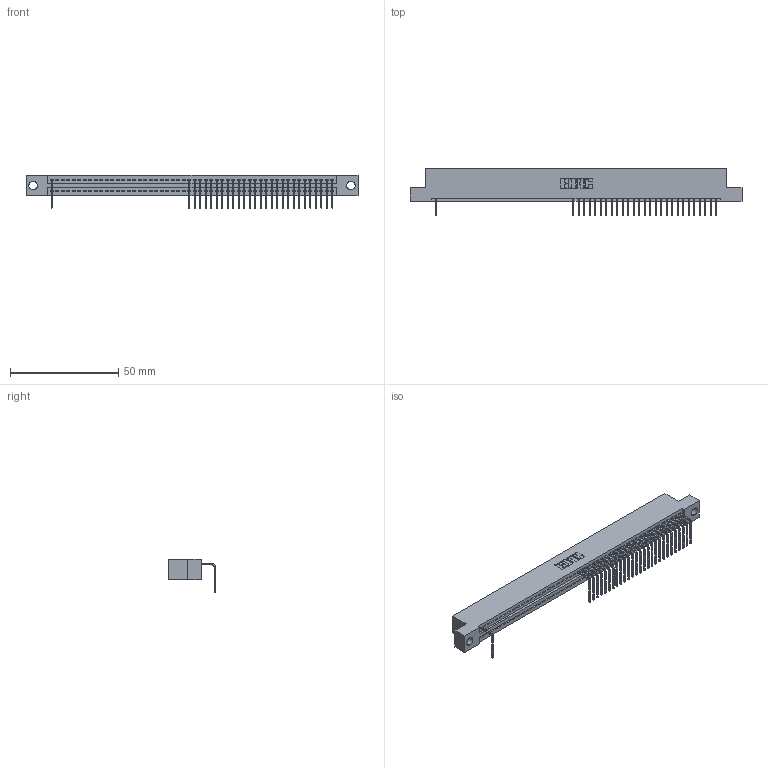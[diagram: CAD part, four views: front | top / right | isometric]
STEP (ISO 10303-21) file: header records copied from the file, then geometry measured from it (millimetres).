
FILE_DESCRIPTION (( 'STEP AP203' ), '1' );
FILE_NAME ('345-052-558-104.STEP', '2018-09-23T00:08:42', ( '' ), ( '' ), 'SwSTEP 2.0', 'SolidWorks 2016', '' );
FILE_SCHEMA (( 'CONFIG_CONTROL_DESIGN' ));
Length unit declared in the file: inch
Products named in the file (3): 345-052-558-104; 345 Part_Flush Mounting Lugs - 0.156 Dia-TH; 345-292-001_558 Tail - 2
Assembly tree (29 placements, depth 2):
  345-052-558-104
    345 Part_Flush Mounting Lugs - 0.156 Dia-TH
    345-292-001_558 Tail - 2  x28
Bounding box: 153.29 x 21.83 x 15.37 mm (x, y, z)
Volume: 14372.1 mm3; surface area: 18132.6 mm2
Topology: 29 solids, 29 shells, 2190 faces, 6733 edges, 4450 vertices
Faces by surface type: plane 1592, cylinder 598
Entity records: 37109 total; most frequent: ORIENTED_EDGE 6554, CARTESIAN_POINT 6544, DIRECTION 5673, EDGE_CURVE 3277, LINE 2937, VECTOR 2937, VERTEX_POINT 2182, AXIS2_PLACEMENT_3D 1368
